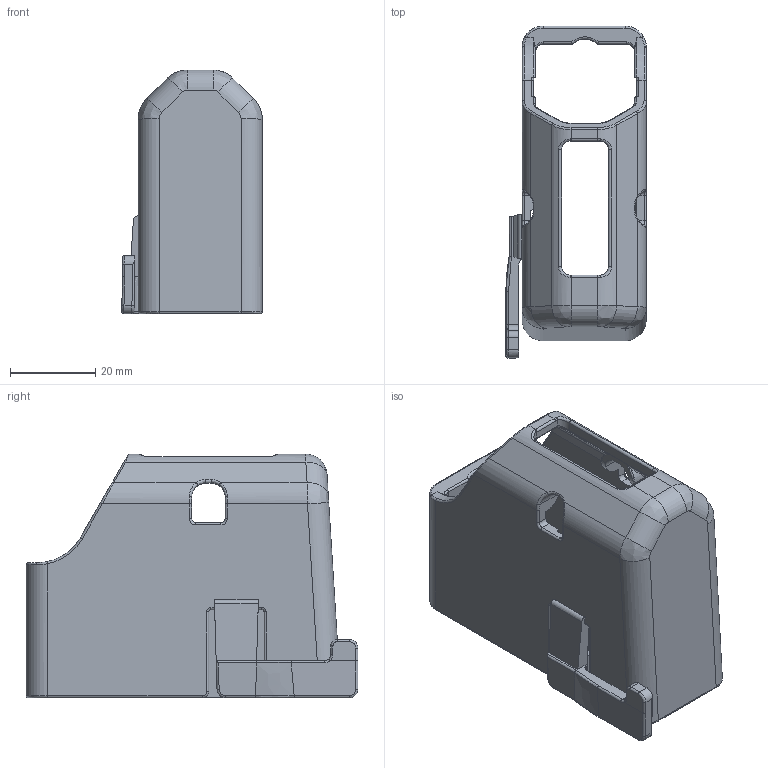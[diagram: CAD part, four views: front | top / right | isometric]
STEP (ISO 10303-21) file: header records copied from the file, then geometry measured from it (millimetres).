
FILE_DESCRIPTION(/* description */ (''),/* implementation_level */ '2;1');
FILE_NAME(/* name */ 'freeloader-body-intergrated-magcatch-plain-v6.step',/* time_stamp */ '2021-09-20T14:46:29-07:00',/* author */ (''),/* organization */ (''),/* preprocessor_version */ 'ST-DEVELOPER v18.1',/* originating_system */ 'Autodesk Translation Framework v10.10.0.1391',/* authorisation */ '');
FILE_SCHEMA (('AUTOMOTIVE_DESIGN { 1 0 10303 214 3 1 1 }'));
Length unit declared in the file: millimetre
Products named in the file (1): loader-base-v2-useThis-plain
Bounding box: 33.05 x 78 x 57.31 mm (x, y, z)
Volume: 28609.5 mm3; surface area: 20686.7 mm2
Topology: 1 solids, 1 shells, 413 faces, 1073 edges, 652 vertices
Faces by surface type: cylinder 142, plane 124, bspline 102, torus 45
Entity records: 15617 total; most frequent: CARTESIAN_POINT 5852, ORIENTED_EDGE 2140, DIRECTION 1943, EDGE_CURVE 1070, AXIS2_PLACEMENT_3D 742, VERTEX_POINT 652, LINE 459, VECTOR 459
